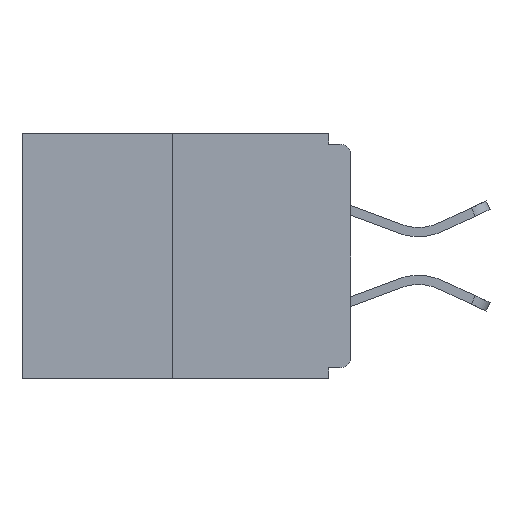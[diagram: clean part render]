
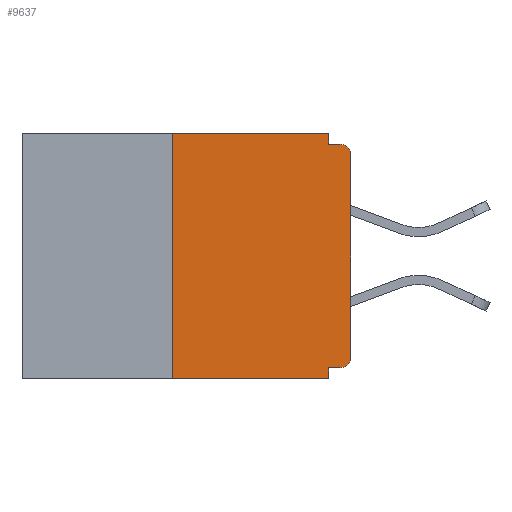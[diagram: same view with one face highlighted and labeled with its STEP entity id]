
A CAD part, left-side view. The second image highlights one B-rep face of the part: STEP entity #9637.
In plain terms, the highlighted planar face has unit normal (-1, 0, 0).
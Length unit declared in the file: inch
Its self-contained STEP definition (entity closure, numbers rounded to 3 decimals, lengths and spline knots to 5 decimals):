
#13 = CARTESIAN_POINT ( 'NONE',  ( 0., 0.031, -0.343 ) ) ;
#381 = DIRECTION ( 'NONE',  ( 0., 0., -1. ) ) ;
#1113 = DIRECTION ( 'NONE',  ( 0., 0., 1. ) ) ;
#1285 = VERTEX_POINT ( 'NONE', #14297 ) ;
#1719 = LINE ( 'NONE', #6906, #25298 ) ;
#1947 = CARTESIAN_POINT ( 'NONE',  ( 0., 0.25, 0. ) ) ;
#2046 = AXIS2_PLACEMENT_3D ( 'NONE', #8112, #5844, #5751 ) ;
#2493 = DIRECTION ( 'NONE',  ( 0., 1., 0. ) ) ;
#2553 = VECTOR ( 'NONE', #381, 39.37008 ) ;
#2587 = VECTOR ( 'NONE', #1113, 39.37008 ) ;
#2702 = DIRECTION ( 'NONE',  ( 1., 0., 0. ) ) ;
#2918 = ORIENTED_EDGE ( 'NONE', *, *, #16435, .F. ) ;
#3190 = LINE ( 'NONE', #4283, #2553 ) ;
#3337 = LINE ( 'NONE', #20994, #6262 ) ;
#4283 = CARTESIAN_POINT ( 'NONE',  ( 0., 0.031, 0. ) ) ;
#4646 = CARTESIAN_POINT ( 'NONE',  ( 0., 0.015, -0.015 ) ) ;
#4731 = CARTESIAN_POINT ( 'NONE',  ( 0., 0.46, -0.343 ) ) ;
#4766 = PLANE ( 'NONE',  #14908 ) ;
#4793 = VECTOR ( 'NONE', #4815, 39.37008 ) ;
#4815 = DIRECTION ( 'NONE',  ( 0., -1., 0. ) ) ;
#5751 = DIRECTION ( 'NONE',  ( 0., 0., -1. ) ) ;
#5844 = DIRECTION ( 'NONE',  ( -1., 0., 0. ) ) ;
#6097 = CARTESIAN_POINT ( 'NONE',  ( 0., 0., -0.03 ) ) ;
#6262 = VECTOR ( 'NONE', #16730, 39.37008 ) ;
#6906 = CARTESIAN_POINT ( 'NONE',  ( 0., 0., -0.015 ) ) ;
#6913 = ORIENTED_EDGE ( 'NONE', *, *, #12901, .F. ) ;
#7372 = ORIENTED_EDGE ( 'NONE', *, *, #25254, .T. ) ;
#7480 = CARTESIAN_POINT ( 'NONE',  ( 0., 0., 0. ) ) ;
#8048 = LINE ( 'NONE', #4731, #4793 ) ;
#8112 = CARTESIAN_POINT ( 'NONE',  ( 0., 0.015, -0.313 ) ) ;
#8501 = VERTEX_POINT ( 'NONE', #10897 ) ;
#8729 = LINE ( 'NONE', #18452, #24526 ) ;
#9082 = CARTESIAN_POINT ( 'NONE',  ( 0., 0.25, -0.343 ) ) ;
#9355 = ORIENTED_EDGE ( 'NONE', *, *, #18072, .F. ) ;
#9545 = CARTESIAN_POINT ( 'NONE',  ( 0., 0., -0.313 ) ) ;
#9637 = ADVANCED_FACE ( 'NONE', ( #24711 ), #4766, .F. ) ;
#10188 = DIRECTION ( 'NONE',  ( -1., 0., 0. ) ) ;
#10278 = ORIENTED_EDGE ( 'NONE', *, *, #13899, .T. ) ;
#10897 = CARTESIAN_POINT ( 'NONE',  ( 0., 0.015, -0.328 ) ) ;
#11189 = VERTEX_POINT ( 'NONE', #4646 ) ;
#12120 = VECTOR ( 'NONE', #14382, 39.37008 ) ;
#12247 = VERTEX_POINT ( 'NONE', #13291 ) ;
#12280 = LINE ( 'NONE', #7480, #2587 ) ;
#12312 = VERTEX_POINT ( 'NONE', #15062 ) ;
#12711 = CARTESIAN_POINT ( 'NONE',  ( 0., 0., -0.328 ) ) ;
#12901 = EDGE_CURVE ( 'NONE', #12312, #1285, #3190, .T. ) ;
#12962 = DIRECTION ( 'NONE',  ( 0., -1., 0. ) ) ;
#12965 = EDGE_CURVE ( 'NONE', #15207, #25509, #8048, .T. ) ;
#13291 = CARTESIAN_POINT ( 'NONE',  ( 0., 0.031, -0.328 ) ) ;
#13899 = EDGE_CURVE ( 'NONE', #16184, #11189, #19863, .T. ) ;
#14297 = CARTESIAN_POINT ( 'NONE',  ( 0., 0.031, -0.015 ) ) ;
#14299 = AXIS2_PLACEMENT_3D ( 'NONE', #22360, #10188, #14402 ) ;
#14382 = DIRECTION ( 'NONE',  ( 0., 0., 1. ) ) ;
#14402 = DIRECTION ( 'NONE',  ( 0., 0., -1. ) ) ;
#14668 = DIRECTION ( 'NONE',  ( 0., 0., -1. ) ) ;
#14908 = AXIS2_PLACEMENT_3D ( 'NONE', #15049, #2702, #26045 ) ;
#15049 = CARTESIAN_POINT ( 'NONE',  ( 0., 0.46, 0. ) ) ;
#15062 = CARTESIAN_POINT ( 'NONE',  ( 0., 0.031, 0. ) ) ;
#15207 = VERTEX_POINT ( 'NONE', #9082 ) ;
#16092 = VERTEX_POINT ( 'NONE', #9545 ) ;
#16184 = VERTEX_POINT ( 'NONE', #6097 ) ;
#16234 = VERTEX_POINT ( 'NONE', #1947 ) ;
#16435 = EDGE_CURVE ( 'NONE', #1285, #11189, #1719, .T. ) ;
#16640 = ORIENTED_EDGE ( 'NONE', *, *, #12965, .T. ) ;
#16730 = DIRECTION ( 'NONE',  ( 0., -1., 0. ) ) ;
#17561 = EDGE_CURVE ( 'NONE', #16092, #16184, #12280, .T. ) ;
#17697 = ORIENTED_EDGE ( 'NONE', *, *, #20008, .F. ) ;
#18072 = EDGE_CURVE ( 'NONE', #12247, #25509, #8729, .T. ) ;
#18452 = CARTESIAN_POINT ( 'NONE',  ( 0., 0.031, -0.343 ) ) ;
#19176 = EDGE_LOOP ( 'NONE', ( #17697, #19749, #16640, #9355, #23185, #7372, #20111, #10278, #2918, #6913 ) ) ;
#19550 = VECTOR ( 'NONE', #2493, 39.37008 ) ;
#19749 = ORIENTED_EDGE ( 'NONE', *, *, #24219, .F. ) ;
#19863 = CIRCLE ( 'NONE', #14299, 0.015 ) ;
#20008 = EDGE_CURVE ( 'NONE', #16234, #12312, #3337, .T. ) ;
#20111 = ORIENTED_EDGE ( 'NONE', *, *, #17561, .T. ) ;
#20994 = CARTESIAN_POINT ( 'NONE',  ( 0., 0.46, 0. ) ) ;
#22360 = CARTESIAN_POINT ( 'NONE',  ( 0., 0.015, -0.03 ) ) ;
#23185 = ORIENTED_EDGE ( 'NONE', *, *, #23642, .F. ) ;
#23642 = EDGE_CURVE ( 'NONE', #8501, #12247, #25085, .T. ) ;
#24219 = EDGE_CURVE ( 'NONE', #15207, #16234, #24389, .T. ) ;
#24389 = LINE ( 'NONE', #24956, #12120 ) ;
#24526 = VECTOR ( 'NONE', #14668, 39.37008 ) ;
#24711 = FACE_OUTER_BOUND ( 'NONE', #19176, .T. ) ;
#24956 = CARTESIAN_POINT ( 'NONE',  ( 0., 0.25, 0. ) ) ;
#24981 = CIRCLE ( 'NONE', #2046, 0.015 ) ;
#25085 = LINE ( 'NONE', #12711, #19550 ) ;
#25254 = EDGE_CURVE ( 'NONE', #8501, #16092, #24981, .T. ) ;
#25298 = VECTOR ( 'NONE', #12962, 39.37008 ) ;
#25509 = VERTEX_POINT ( 'NONE', #13 ) ;
#26045 = DIRECTION ( 'NONE',  ( 0., 0., -1. ) ) ;
